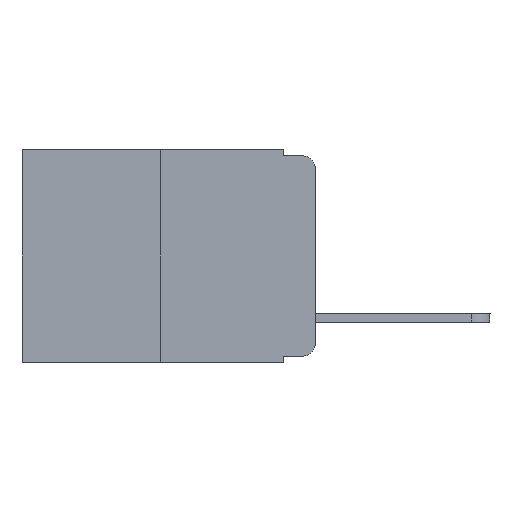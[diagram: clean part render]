
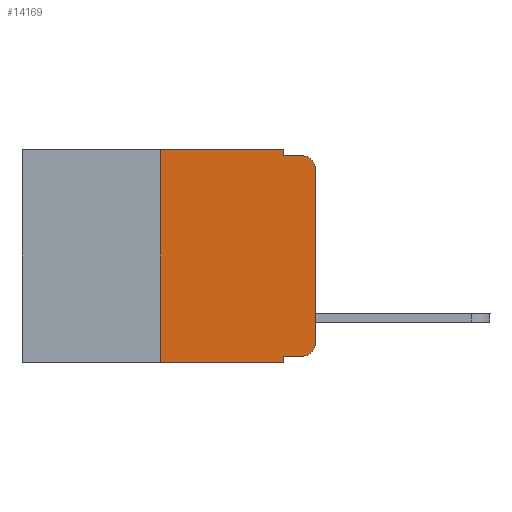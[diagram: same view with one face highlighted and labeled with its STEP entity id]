
A CAD part, left-side view. The second image highlights one B-rep face of the part: STEP entity #14169.
In plain terms, the highlighted planar face has unit normal (-1, 0, 0).
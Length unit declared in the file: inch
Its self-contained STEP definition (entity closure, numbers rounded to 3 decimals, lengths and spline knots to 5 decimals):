
#574 = CARTESIAN_POINT ( 'NONE',  ( 0., 0.02, -0.333 ) ) ;
#756 = CARTESIAN_POINT ( 'NONE',  ( 0., 0.051, -0.333 ) ) ;
#764 = ORIENTED_EDGE ( 'NONE', *, *, #8000, .T. ) ;
#1005 = ORIENTED_EDGE ( 'NONE', *, *, #1106, .F. ) ;
#1051 = ORIENTED_EDGE ( 'NONE', *, *, #20379, .F. ) ;
#1102 = DIRECTION ( 'NONE',  ( 0., 0., -1. ) ) ;
#1106 = EDGE_CURVE ( 'NONE', #3097, #4632, #18258, .T. ) ;
#1159 = DIRECTION ( 'NONE',  ( 0., 0., -1. ) ) ;
#1526 = EDGE_CURVE ( 'NONE', #19142, #4632, #2105, .T. ) ;
#1671 = VERTEX_POINT ( 'NONE', #9491 ) ;
#1791 = VECTOR ( 'NONE', #15103, 39.37008 ) ;
#2105 = LINE ( 'NONE', #15688, #20307 ) ;
#2128 = CARTESIAN_POINT ( 'NONE',  ( 0., 0.25, -0.343 ) ) ;
#2179 = AXIS2_PLACEMENT_3D ( 'NONE', #14143, #17477, #22645 ) ;
#2202 = CARTESIAN_POINT ( 'NONE',  ( 0., 0.02, -0.01 ) ) ;
#2784 = CARTESIAN_POINT ( 'NONE',  ( 0., 0.02, -0.03 ) ) ;
#3084 = CARTESIAN_POINT ( 'NONE',  ( 0., 0.02, -0.313 ) ) ;
#3097 = VERTEX_POINT ( 'NONE', #20215 ) ;
#3143 = AXIS2_PLACEMENT_3D ( 'NONE', #3084, #15425, #4865 ) ;
#3337 = ORIENTED_EDGE ( 'NONE', *, *, #20304, .T. ) ;
#3704 = ORIENTED_EDGE ( 'NONE', *, *, #9426, .F. ) ;
#3986 = LINE ( 'NONE', #22134, #4826 ) ;
#4262 = VERTEX_POINT ( 'NONE', #7450 ) ;
#4488 = CIRCLE ( 'NONE', #19430, 0.02 ) ;
#4632 = VERTEX_POINT ( 'NONE', #22551 ) ;
#4679 = VECTOR ( 'NONE', #9195, 39.37008 ) ;
#4726 = CARTESIAN_POINT ( 'NONE',  ( 0., 0.051, 0. ) ) ;
#4826 = VECTOR ( 'NONE', #10250, 39.37008 ) ;
#4865 = DIRECTION ( 'NONE',  ( 0., 0., -1. ) ) ;
#5451 = ORIENTED_EDGE ( 'NONE', *, *, #1526, .T. ) ;
#7450 = CARTESIAN_POINT ( 'NONE',  ( 0., 0., -0.03 ) ) ;
#7535 = EDGE_LOOP ( 'NONE', ( #9634, #19963, #1051, #19203, #3704, #21301, #5451, #1005, #3337, #764 ) ) ;
#8000 = EDGE_CURVE ( 'NONE', #16175, #11233, #19343, .T. ) ;
#8634 = PLANE ( 'NONE',  #2179 ) ;
#9043 = CARTESIAN_POINT ( 'NONE',  ( 0., 0.473, 0. ) ) ;
#9195 = DIRECTION ( 'NONE',  ( 0., -1., 0. ) ) ;
#9426 = EDGE_CURVE ( 'NONE', #1671, #15384, #18755, .T. ) ;
#9491 = CARTESIAN_POINT ( 'NONE',  ( 0., 0.25, 0. ) ) ;
#9634 = ORIENTED_EDGE ( 'NONE', *, *, #20091, .T. ) ;
#9857 = DIRECTION ( 'NONE',  ( 0., 0., 1. ) ) ;
#10250 = DIRECTION ( 'NONE',  ( 0., -1., 0. ) ) ;
#10393 = DIRECTION ( 'NONE',  ( 0., 0., -1. ) ) ;
#10494 = CARTESIAN_POINT ( 'NONE',  ( 0., 0.051, 0. ) ) ;
#10577 = CARTESIAN_POINT ( 'NONE',  ( 0., 0.051, -0.01 ) ) ;
#10960 = VECTOR ( 'NONE', #9857, 39.37008 ) ;
#11108 = CARTESIAN_POINT ( 'NONE',  ( 0., 0., 0. ) ) ;
#11233 = VERTEX_POINT ( 'NONE', #18591 ) ;
#11308 = FACE_OUTER_BOUND ( 'NONE', #7535, .T. ) ;
#11607 = DIRECTION ( 'NONE',  ( -1., 0., 0. ) ) ;
#11838 = VERTEX_POINT ( 'NONE', #2202 ) ;
#11947 = EDGE_CURVE ( 'NONE', #19142, #1671, #15640, .T. ) ;
#12581 = VECTOR ( 'NONE', #10393, 39.37008 ) ;
#13585 = VECTOR ( 'NONE', #1102, 39.37008 ) ;
#13918 = DIRECTION ( 'NONE',  ( 0., -1., 0. ) ) ;
#14143 = CARTESIAN_POINT ( 'NONE',  ( 0., 0.473, 0. ) ) ;
#14169 = ADVANCED_FACE ( 'NONE', ( #11308 ), #8634, .F. ) ;
#15103 = DIRECTION ( 'NONE',  ( 0., -1., 0. ) ) ;
#15384 = VERTEX_POINT ( 'NONE', #10494 ) ;
#15425 = DIRECTION ( 'NONE',  ( -1., 0., 0. ) ) ;
#15640 = LINE ( 'NONE', #18474, #10960 ) ;
#15688 = CARTESIAN_POINT ( 'NONE',  ( 0., 0.473, -0.343 ) ) ;
#15957 = VECTOR ( 'NONE', #17955, 39.37008 ) ;
#15958 = EDGE_CURVE ( 'NONE', #15384, #22458, #16457, .T. ) ;
#16175 = VERTEX_POINT ( 'NONE', #574 ) ;
#16457 = LINE ( 'NONE', #20899, #12581 ) ;
#17477 = DIRECTION ( 'NONE',  ( 1., 0., 0. ) ) ;
#17955 = DIRECTION ( 'NONE',  ( 0., 0., 1. ) ) ;
#18157 = LINE ( 'NONE', #11108, #15957 ) ;
#18258 = LINE ( 'NONE', #4726, #13585 ) ;
#18474 = CARTESIAN_POINT ( 'NONE',  ( 0., 0.25, 0. ) ) ;
#18591 = CARTESIAN_POINT ( 'NONE',  ( 0., 0., -0.313 ) ) ;
#18755 = LINE ( 'NONE', #9043, #4679 ) ;
#19142 = VERTEX_POINT ( 'NONE', #2128 ) ;
#19203 = ORIENTED_EDGE ( 'NONE', *, *, #15958, .F. ) ;
#19343 = CIRCLE ( 'NONE', #3143, 0.02 ) ;
#19430 = AXIS2_PLACEMENT_3D ( 'NONE', #2784, #11607, #1159 ) ;
#19963 = ORIENTED_EDGE ( 'NONE', *, *, #21442, .T. ) ;
#20091 = EDGE_CURVE ( 'NONE', #11233, #4262, #18157, .T. ) ;
#20215 = CARTESIAN_POINT ( 'NONE',  ( 0., 0.051, -0.333 ) ) ;
#20304 = EDGE_CURVE ( 'NONE', #3097, #16175, #21881, .T. ) ;
#20307 = VECTOR ( 'NONE', #13918, 39.37008 ) ;
#20379 = EDGE_CURVE ( 'NONE', #22458, #11838, #3986, .T. ) ;
#20899 = CARTESIAN_POINT ( 'NONE',  ( 0., 0.051, 0. ) ) ;
#21301 = ORIENTED_EDGE ( 'NONE', *, *, #11947, .F. ) ;
#21442 = EDGE_CURVE ( 'NONE', #4262, #11838, #4488, .T. ) ;
#21881 = LINE ( 'NONE', #756, #1791 ) ;
#22134 = CARTESIAN_POINT ( 'NONE',  ( 0., 0.051, -0.01 ) ) ;
#22458 = VERTEX_POINT ( 'NONE', #10577 ) ;
#22551 = CARTESIAN_POINT ( 'NONE',  ( 0., 0.051, -0.343 ) ) ;
#22645 = DIRECTION ( 'NONE',  ( 0., 0., -1. ) ) ;
